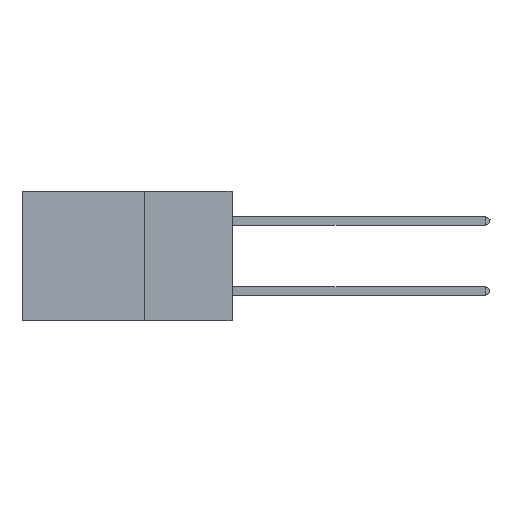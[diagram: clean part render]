
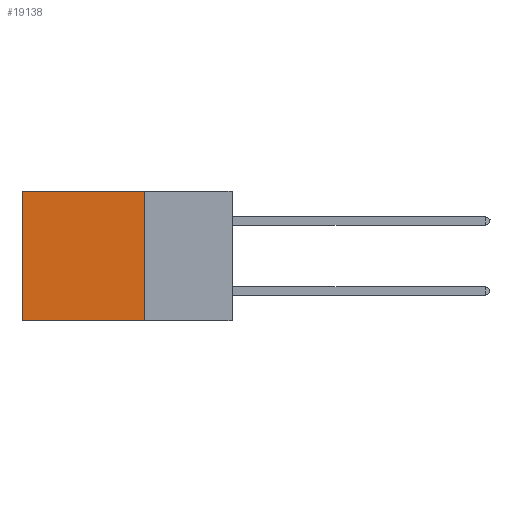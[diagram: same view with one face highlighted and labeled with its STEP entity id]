
A CAD part, left-side view. The second image highlights one B-rep face of the part: STEP entity #19138.
In plain terms, the highlighted planar face has unit normal (-1, 0, 0).
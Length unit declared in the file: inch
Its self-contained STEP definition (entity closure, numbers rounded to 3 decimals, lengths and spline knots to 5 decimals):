
#600 = EDGE_CURVE ( 'NONE', #7864, #9390, #35560, .T. ) ;
#1594 = DIRECTION ( 'NONE',  ( 0., 1., 0. ) ) ;
#3762 = EDGE_CURVE ( 'NONE', #7864, #27056, #21349, .T. ) ;
#3834 = CARTESIAN_POINT ( 'NONE',  ( 0.2875, 0.25, 0. ) ) ;
#5508 = CARTESIAN_POINT ( 'NONE',  ( 0.2875, 0.25, -0.37 ) ) ;
#7864 = VERTEX_POINT ( 'NONE', #43126 ) ;
#7890 = CARTESIAN_POINT ( 'NONE',  ( 0.2875, 0.25, 0. ) ) ;
#7931 = LINE ( 'NONE', #18155, #37747 ) ;
#9390 = VERTEX_POINT ( 'NONE', #19239 ) ;
#12012 = VECTOR ( 'NONE', #1594, 39.37008 ) ;
#14338 = DIRECTION ( 'NONE',  ( 0., 1., 0. ) ) ;
#15451 = CARTESIAN_POINT ( 'NONE',  ( 0.2875, 0.6, -0.37 ) ) ;
#16995 = CARTESIAN_POINT ( 'NONE',  ( 0.2875, 0.25, 0. ) ) ;
#17719 = DIRECTION ( 'NONE',  ( 0., 0., -1. ) ) ;
#18155 = CARTESIAN_POINT ( 'NONE',  ( 0.2875, 0.6, 0. ) ) ;
#18516 = ORIENTED_EDGE ( 'NONE', *, *, #600, .T. ) ;
#19138 = ADVANCED_FACE ( 'NONE', ( #27146 ), #23690, .F. ) ;
#19239 = CARTESIAN_POINT ( 'NONE',  ( 0.2875, 0.6, 0. ) ) ;
#21349 = LINE ( 'NONE', #3834, #31432 ) ;
#21550 = EDGE_LOOP ( 'NONE', ( #22806, #30351, #27734, #18516 ) ) ;
#22806 = ORIENTED_EDGE ( 'NONE', *, *, #35617, .T. ) ;
#23479 = LINE ( 'NONE', #5508, #12012 ) ;
#23690 = PLANE ( 'NONE',  #43314 ) ;
#27056 = VERTEX_POINT ( 'NONE', #33844 ) ;
#27146 = FACE_OUTER_BOUND ( 'NONE', #21550, .T. ) ;
#27380 = DIRECTION ( 'NONE',  ( 0., 0., -1. ) ) ;
#27734 = ORIENTED_EDGE ( 'NONE', *, *, #3762, .F. ) ;
#30351 = ORIENTED_EDGE ( 'NONE', *, *, #41896, .F. ) ;
#31432 = VECTOR ( 'NONE', #31956, 39.37008 ) ;
#31956 = DIRECTION ( 'NONE',  ( 0., 0., -1. ) ) ;
#33844 = CARTESIAN_POINT ( 'NONE',  ( 0.2875, 0.25, -0.37 ) ) ;
#35560 = LINE ( 'NONE', #7890, #43010 ) ;
#35617 = EDGE_CURVE ( 'NONE', #9390, #40805, #7931, .T. ) ;
#37747 = VECTOR ( 'NONE', #17719, 39.37008 ) ;
#40774 = DIRECTION ( 'NONE',  ( 1., 0., 0. ) ) ;
#40805 = VERTEX_POINT ( 'NONE', #15451 ) ;
#41896 = EDGE_CURVE ( 'NONE', #27056, #40805, #23479, .T. ) ;
#43010 = VECTOR ( 'NONE', #14338, 39.37008 ) ;
#43126 = CARTESIAN_POINT ( 'NONE',  ( 0.2875, 0.25, 0. ) ) ;
#43314 = AXIS2_PLACEMENT_3D ( 'NONE', #16995, #40774, #27380 ) ;
